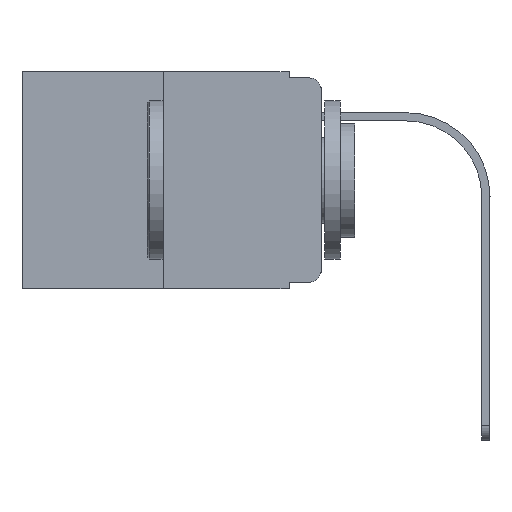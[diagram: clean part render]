
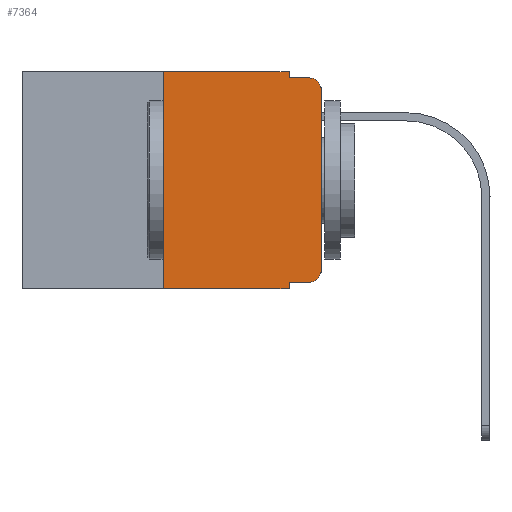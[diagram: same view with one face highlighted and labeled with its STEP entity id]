
A CAD part, left-side view. The second image highlights one B-rep face of the part: STEP entity #7364.
In plain terms, the highlighted planar face has unit normal (-1, 0, 0).
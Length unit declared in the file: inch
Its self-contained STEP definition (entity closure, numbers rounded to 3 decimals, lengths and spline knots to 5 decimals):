
#435 = EDGE_CURVE ( 'NONE', #1115, #16506, #8350, .T. ) ;
#710 = VECTOR ( 'NONE', #8253, 39.37008 ) ;
#1115 = VERTEX_POINT ( 'NONE', #1265 ) ;
#1265 = CARTESIAN_POINT ( 'NONE',  ( 0., 0.051, -0.01 ) ) ;
#1790 = CARTESIAN_POINT ( 'NONE',  ( 0., 0.051, -0.333 ) ) ;
#1956 = DIRECTION ( 'NONE',  ( 0., 0., -1. ) ) ;
#1979 = VECTOR ( 'NONE', #10881, 39.37008 ) ;
#2282 = CARTESIAN_POINT ( 'NONE',  ( 0., 0.051, 0. ) ) ;
#2318 = VECTOR ( 'NONE', #13960, 39.37008 ) ;
#2367 = EDGE_CURVE ( 'NONE', #13496, #10369, #5277, .T. ) ;
#2410 = DIRECTION ( 'NONE',  ( 0., 0., -1. ) ) ;
#2883 = ORIENTED_EDGE ( 'NONE', *, *, #2367, .T. ) ;
#2996 = VERTEX_POINT ( 'NONE', #10276 ) ;
#3166 = DIRECTION ( 'NONE',  ( 0., -1., 0. ) ) ;
#3361 = VECTOR ( 'NONE', #3166, 39.37008 ) ;
#3443 = VERTEX_POINT ( 'NONE', #10063 ) ;
#3543 = EDGE_CURVE ( 'NONE', #13439, #17697, #17397, .T. ) ;
#4337 = VECTOR ( 'NONE', #6469, 39.37008 ) ;
#4701 = EDGE_CURVE ( 'NONE', #10369, #16506, #7069, .T. ) ;
#4756 = DIRECTION ( 'NONE',  ( -1., 0., 0. ) ) ;
#4771 = PLANE ( 'NONE',  #14850 ) ;
#5039 = CARTESIAN_POINT ( 'NONE',  ( 0., 0.473, -0.343 ) ) ;
#5178 = DIRECTION ( 'NONE',  ( 0., 0., -1. ) ) ;
#5277 = LINE ( 'NONE', #9330, #1979 ) ;
#5486 = CARTESIAN_POINT ( 'NONE',  ( 0., 0.051, -0.343 ) ) ;
#5664 = CARTESIAN_POINT ( 'NONE',  ( 0., 0.051, -0.333 ) ) ;
#5845 = ORIENTED_EDGE ( 'NONE', *, *, #3543, .F. ) ;
#6469 = DIRECTION ( 'NONE',  ( 0., 0., 1. ) ) ;
#6508 = VERTEX_POINT ( 'NONE', #16154 ) ;
#6635 = EDGE_CURVE ( 'NONE', #3443, #17697, #16628, .T. ) ;
#6935 = CIRCLE ( 'NONE', #12511, 0.02 ) ;
#7069 = CIRCLE ( 'NONE', #12940, 0.02 ) ;
#7319 = CARTESIAN_POINT ( 'NONE',  ( 0., 0.25, 0. ) ) ;
#7364 = ADVANCED_FACE ( 'NONE', ( #17453 ), #4771, .F. ) ;
#7711 = DIRECTION ( 'NONE',  ( 1., 0., 0. ) ) ;
#7712 = ORIENTED_EDGE ( 'NONE', *, *, #12903, .F. ) ;
#7878 = CARTESIAN_POINT ( 'NONE',  ( 0., 0.02, -0.01 ) ) ;
#7923 = ORIENTED_EDGE ( 'NONE', *, *, #14911, .F. ) ;
#7997 = ORIENTED_EDGE ( 'NONE', *, *, #8157, .T. ) ;
#8157 = EDGE_CURVE ( 'NONE', #13439, #2996, #16791, .T. ) ;
#8253 = DIRECTION ( 'NONE',  ( 0., -1., 0. ) ) ;
#8350 = LINE ( 'NONE', #11193, #710 ) ;
#8560 = EDGE_LOOP ( 'NONE', ( #2883, #13843, #11122, #15404, #7923, #7712, #17018, #5845, #7997, #11983 ) ) ;
#8637 = CARTESIAN_POINT ( 'NONE',  ( 0., 0.02, -0.313 ) ) ;
#8806 = CARTESIAN_POINT ( 'NONE',  ( 0., 0., -0.313 ) ) ;
#8837 = LINE ( 'NONE', #10476, #3361 ) ;
#9327 = DIRECTION ( 'NONE',  ( -1., 0., 0. ) ) ;
#9330 = CARTESIAN_POINT ( 'NONE',  ( 0., 0., 0. ) ) ;
#9458 = CARTESIAN_POINT ( 'NONE',  ( 0., 0., -0.03 ) ) ;
#9709 = LINE ( 'NONE', #10830, #4337 ) ;
#10063 = CARTESIAN_POINT ( 'NONE',  ( 0., 0.25, -0.343 ) ) ;
#10276 = CARTESIAN_POINT ( 'NONE',  ( 0., 0.02, -0.333 ) ) ;
#10369 = VERTEX_POINT ( 'NONE', #9458 ) ;
#10476 = CARTESIAN_POINT ( 'NONE',  ( 0., 0.473, 0. ) ) ;
#10493 = VECTOR ( 'NONE', #11277, 39.37008 ) ;
#10544 = VERTEX_POINT ( 'NONE', #7319 ) ;
#10698 = CARTESIAN_POINT ( 'NONE',  ( 0., 0.02, -0.03 ) ) ;
#10801 = DIRECTION ( 'NONE',  ( 0., 0., -1. ) ) ;
#10830 = CARTESIAN_POINT ( 'NONE',  ( 0., 0.25, 0. ) ) ;
#10881 = DIRECTION ( 'NONE',  ( 0., 0., 1. ) ) ;
#11122 = ORIENTED_EDGE ( 'NONE', *, *, #435, .F. ) ;
#11193 = CARTESIAN_POINT ( 'NONE',  ( 0., 0.051, -0.01 ) ) ;
#11277 = DIRECTION ( 'NONE',  ( 0., -1., 0. ) ) ;
#11861 = EDGE_CURVE ( 'NONE', #6508, #1115, #16655, .T. ) ;
#11983 = ORIENTED_EDGE ( 'NONE', *, *, #12771, .T. ) ;
#12326 = CARTESIAN_POINT ( 'NONE',  ( 0., 0.051, 0. ) ) ;
#12511 = AXIS2_PLACEMENT_3D ( 'NONE', #8637, #4756, #1956 ) ;
#12771 = EDGE_CURVE ( 'NONE', #2996, #13496, #6935, .T. ) ;
#12903 = EDGE_CURVE ( 'NONE', #3443, #10544, #9709, .T. ) ;
#12940 = AXIS2_PLACEMENT_3D ( 'NONE', #10698, #9327, #5178 ) ;
#13439 = VERTEX_POINT ( 'NONE', #1790 ) ;
#13496 = VERTEX_POINT ( 'NONE', #8806 ) ;
#13843 = ORIENTED_EDGE ( 'NONE', *, *, #4701, .T. ) ;
#13960 = DIRECTION ( 'NONE',  ( 0., 0., -1. ) ) ;
#14479 = VECTOR ( 'NONE', #10801, 39.37008 ) ;
#14760 = CARTESIAN_POINT ( 'NONE',  ( 0., 0.473, 0. ) ) ;
#14768 = DIRECTION ( 'NONE',  ( 0., -1., 0. ) ) ;
#14850 = AXIS2_PLACEMENT_3D ( 'NONE', #14760, #7711, #2410 ) ;
#14911 = EDGE_CURVE ( 'NONE', #10544, #6508, #8837, .T. ) ;
#15318 = VECTOR ( 'NONE', #14768, 39.37008 ) ;
#15404 = ORIENTED_EDGE ( 'NONE', *, *, #11861, .F. ) ;
#16154 = CARTESIAN_POINT ( 'NONE',  ( 0., 0.051, 0. ) ) ;
#16506 = VERTEX_POINT ( 'NONE', #7878 ) ;
#16628 = LINE ( 'NONE', #5039, #15318 ) ;
#16655 = LINE ( 'NONE', #12326, #2318 ) ;
#16791 = LINE ( 'NONE', #5664, #10493 ) ;
#17018 = ORIENTED_EDGE ( 'NONE', *, *, #6635, .T. ) ;
#17397 = LINE ( 'NONE', #2282, #14479 ) ;
#17453 = FACE_OUTER_BOUND ( 'NONE', #8560, .T. ) ;
#17697 = VERTEX_POINT ( 'NONE', #5486 ) ;
